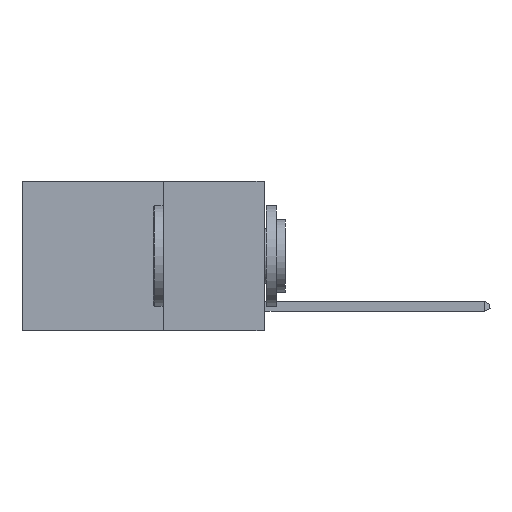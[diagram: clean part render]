
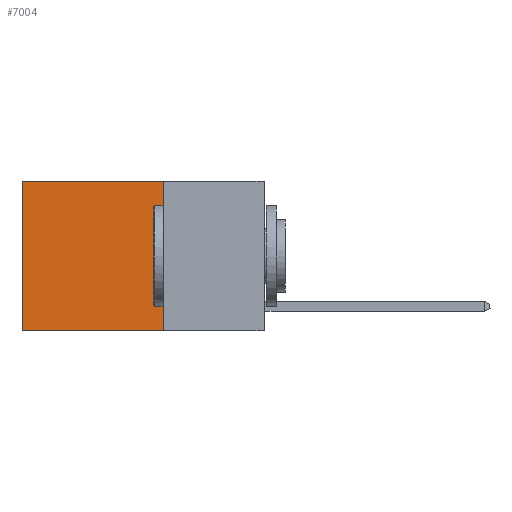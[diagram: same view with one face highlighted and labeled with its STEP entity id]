
A CAD part, left-side view. The second image highlights one B-rep face of the part: STEP entity #7004.
In plain terms, the highlighted planar face has unit normal (-1, 0, 0).
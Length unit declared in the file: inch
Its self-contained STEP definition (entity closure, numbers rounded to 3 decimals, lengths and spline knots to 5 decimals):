
#71 = CARTESIAN_POINT ( 'NONE',  ( 0.2625, 0.6, 0. ) ) ;
#260 = CARTESIAN_POINT ( 'NONE',  ( 0.2625, 0.6, 0. ) ) ;
#561 = PLANE ( 'NONE',  #12172 ) ;
#814 = CARTESIAN_POINT ( 'NONE',  ( 0.2625, 0.25, -0.37 ) ) ;
#1454 = ORIENTED_EDGE ( 'NONE', *, *, #9321, .F. ) ;
#1599 = CARTESIAN_POINT ( 'NONE',  ( 0.2625, 0.25, 0. ) ) ;
#1774 = FACE_OUTER_BOUND ( 'NONE', #3935, .T. ) ;
#2492 = VECTOR ( 'NONE', #3688, 39.37008 ) ;
#3012 = EDGE_CURVE ( 'NONE', #9622, #9073, #12721, .T. ) ;
#3186 = VECTOR ( 'NONE', #7374, 39.37008 ) ;
#3533 = LINE ( 'NONE', #15002, #2492 ) ;
#3570 = ORIENTED_EDGE ( 'NONE', *, *, #3012, .T. ) ;
#3688 = DIRECTION ( 'NONE',  ( 0., 1., 0. ) ) ;
#3935 = EDGE_LOOP ( 'NONE', ( #3570, #9498, #1454, #10909 ) ) ;
#4205 = CARTESIAN_POINT ( 'NONE',  ( 0.2625, 0.6, -0.37 ) ) ;
#6383 = VECTOR ( 'NONE', #11339, 39.37008 ) ;
#7004 = ADVANCED_FACE ( 'NONE', ( #1774 ), #561, .F. ) ;
#7374 = DIRECTION ( 'NONE',  ( 0., 0., -1. ) ) ;
#8164 = DIRECTION ( 'NONE',  ( 0., 0., -1. ) ) ;
#8753 = EDGE_CURVE ( 'NONE', #14494, #9622, #3533, .T. ) ;
#9073 = VERTEX_POINT ( 'NONE', #4205 ) ;
#9321 = EDGE_CURVE ( 'NONE', #14494, #11499, #14303, .T. ) ;
#9494 = CARTESIAN_POINT ( 'NONE',  ( 0.2625, 0.25, 0. ) ) ;
#9498 = ORIENTED_EDGE ( 'NONE', *, *, #11107, .F. ) ;
#9622 = VERTEX_POINT ( 'NONE', #71 ) ;
#9710 = CARTESIAN_POINT ( 'NONE',  ( 0.2625, 0.25, 0. ) ) ;
#9849 = DIRECTION ( 'NONE',  ( 0., 0., -1. ) ) ;
#9956 = LINE ( 'NONE', #814, #6383 ) ;
#10909 = ORIENTED_EDGE ( 'NONE', *, *, #8753, .T. ) ;
#11107 = EDGE_CURVE ( 'NONE', #11499, #9073, #9956, .T. ) ;
#11339 = DIRECTION ( 'NONE',  ( 0., 1., 0. ) ) ;
#11499 = VERTEX_POINT ( 'NONE', #12371 ) ;
#12070 = DIRECTION ( 'NONE',  ( 1., 0., 0. ) ) ;
#12172 = AXIS2_PLACEMENT_3D ( 'NONE', #9710, #12070, #9849 ) ;
#12371 = CARTESIAN_POINT ( 'NONE',  ( 0.2625, 0.25, -0.37 ) ) ;
#12721 = LINE ( 'NONE', #260, #14534 ) ;
#14303 = LINE ( 'NONE', #1599, #3186 ) ;
#14494 = VERTEX_POINT ( 'NONE', #9494 ) ;
#14534 = VECTOR ( 'NONE', #8164, 39.37008 ) ;
#15002 = CARTESIAN_POINT ( 'NONE',  ( 0.2625, 0.25, 0. ) ) ;
